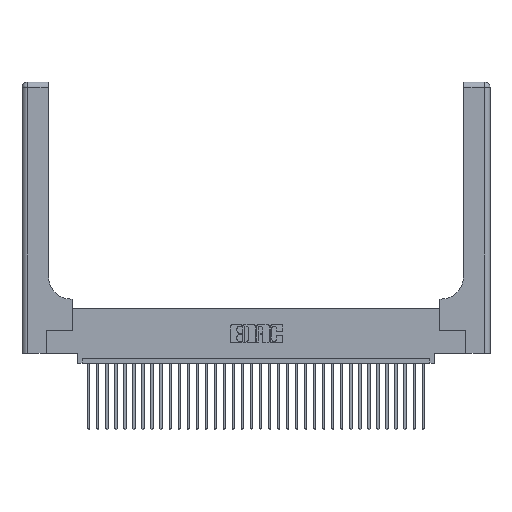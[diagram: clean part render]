
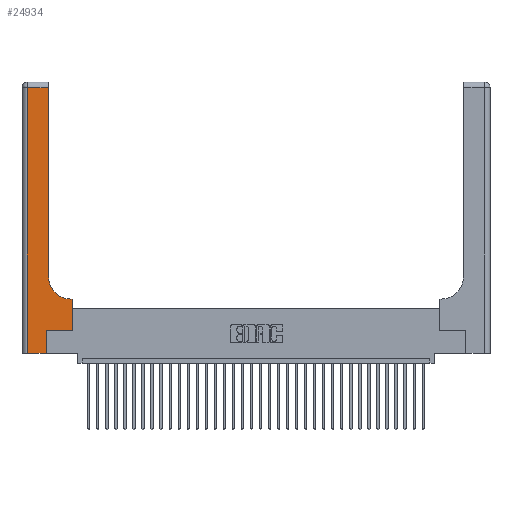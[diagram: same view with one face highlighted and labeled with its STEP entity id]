
A CAD part, top view. The second image highlights one B-rep face of the part: STEP entity #24934.
In plain terms, the highlighted planar face has unit normal (0, 0, 1).
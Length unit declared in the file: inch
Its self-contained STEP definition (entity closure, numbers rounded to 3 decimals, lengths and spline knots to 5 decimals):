
#154 = EDGE_CURVE ( 'NONE', #21570, #16127, #9224, .T. ) ;
#221 = DIRECTION ( 'NONE',  ( 1., 0., 0. ) ) ;
#1286 = CARTESIAN_POINT ( 'NONE',  ( 0.5585, 0.25, 0.37 ) ) ;
#1710 = DIRECTION ( 'NONE',  ( 0., -1., 0. ) ) ;
#2598 = LINE ( 'NONE', #5980, #32109 ) ;
#3594 = EDGE_CURVE ( 'NONE', #24266, #9584, #24757, .T. ) ;
#4675 = ORIENTED_EDGE ( 'NONE', *, *, #27138, .T. ) ;
#5340 = CARTESIAN_POINT ( 'NONE',  ( 0.269, 0.25, 0.37 ) ) ;
#5580 = CARTESIAN_POINT ( 'NONE',  ( 0.5415, 0.85, 0.37 ) ) ;
#5738 = VECTOR ( 'NONE', #5761, 39.37008 ) ;
#5761 = DIRECTION ( 'NONE',  ( 1., 0., 0. ) ) ;
#5980 = CARTESIAN_POINT ( 'NONE',  ( 0., 2.94, 0.37 ) ) ;
#6975 = VECTOR ( 'NONE', #34010, 39.37008 ) ;
#7863 = ORIENTED_EDGE ( 'NONE', *, *, #18784, .T. ) ;
#8684 = AXIS2_PLACEMENT_3D ( 'NONE', #11112, #29748, #29986 ) ;
#8697 = DIRECTION ( 'NONE',  ( 0., 0., -1. ) ) ;
#8707 = EDGE_CURVE ( 'NONE', #16127, #24266, #9422, .T. ) ;
#8940 = ORIENTED_EDGE ( 'NONE', *, *, #33445, .T. ) ;
#9014 = AXIS2_PLACEMENT_3D ( 'NONE', #5580, #8697, #221 ) ;
#9154 = CARTESIAN_POINT ( 'NONE',  ( 0.269, 0., 0.37 ) ) ;
#9224 = LINE ( 'NONE', #1286, #30463 ) ;
#9422 = LINE ( 'NONE', #27521, #29785 ) ;
#9584 = VERTEX_POINT ( 'NONE', #18418 ) ;
#11112 = CARTESIAN_POINT ( 'NONE',  ( 0., 3., 0.37 ) ) ;
#11221 = ORIENTED_EDGE ( 'NONE', *, *, #30206, .T. ) ;
#11396 = CARTESIAN_POINT ( 'NONE',  ( 0.5415, 0.6, 0.37 ) ) ;
#11425 = DIRECTION ( 'NONE',  ( -1., 0., 0. ) ) ;
#11438 = CARTESIAN_POINT ( 'NONE',  ( 0.2915, 2.94, 0.37 ) ) ;
#13589 = CARTESIAN_POINT ( 'NONE',  ( 0.2915, 3., 0.37 ) ) ;
#13590 = EDGE_CURVE ( 'NONE', #15909, #21570, #17834, .T. ) ;
#13666 = CARTESIAN_POINT ( 'NONE',  ( 0.269, 0.25, 0.37 ) ) ;
#14011 = LINE ( 'NONE', #13589, #6975 ) ;
#15769 = DIRECTION ( 'NONE',  ( 0., 1., 0. ) ) ;
#15810 = CARTESIAN_POINT ( 'NONE',  ( 0.06, 0., 0.37 ) ) ;
#15909 = VERTEX_POINT ( 'NONE', #5340 ) ;
#16071 = ORIENTED_EDGE ( 'NONE', *, *, #154, .T. ) ;
#16127 = VERTEX_POINT ( 'NONE', #21153 ) ;
#16773 = DIRECTION ( 'NONE',  ( -1., 0., 0. ) ) ;
#17480 = ORIENTED_EDGE ( 'NONE', *, *, #13590, .T. ) ;
#17834 = LINE ( 'NONE', #13666, #5738 ) ;
#18418 = CARTESIAN_POINT ( 'NONE',  ( 0.2915, 0.85, 0.37 ) ) ;
#18691 = CARTESIAN_POINT ( 'NONE',  ( 0.5585, 0.25, 0.37 ) ) ;
#18784 = EDGE_CURVE ( 'NONE', #23771, #28457, #2598, .T. ) ;
#19118 = VECTOR ( 'NONE', #15769, 39.37008 ) ;
#20869 = EDGE_CURVE ( 'NONE', #28652, #15909, #32092, .T. ) ;
#21153 = CARTESIAN_POINT ( 'NONE',  ( 0.5585, 0.6, 0.37 ) ) ;
#21570 = VERTEX_POINT ( 'NONE', #18691 ) ;
#22500 = EDGE_LOOP ( 'NONE', ( #8940, #7863, #11221, #4675, #31998, #17480, #16071, #22755, #31070 ) ) ;
#22755 = ORIENTED_EDGE ( 'NONE', *, *, #8707, .T. ) ;
#23032 = CARTESIAN_POINT ( 'NONE',  ( 0.06, 3., 0.37 ) ) ;
#23771 = VERTEX_POINT ( 'NONE', #11438 ) ;
#24266 = VERTEX_POINT ( 'NONE', #11396 ) ;
#24439 = CARTESIAN_POINT ( 'NONE',  ( 0.06, 2.94, 0.37 ) ) ;
#24736 = VERTEX_POINT ( 'NONE', #15810 ) ;
#24757 = CIRCLE ( 'NONE', #9014, 0.25 ) ;
#24934 = ADVANCED_FACE ( 'NONE', ( #29692 ), #27300, .F. ) ;
#25077 = DIRECTION ( 'NONE',  ( 0., 1., 0. ) ) ;
#26659 = CARTESIAN_POINT ( 'NONE',  ( 0., 0., 0.37 ) ) ;
#26871 = VECTOR ( 'NONE', #1710, 39.37008 ) ;
#27138 = EDGE_CURVE ( 'NONE', #24736, #28652, #32529, .T. ) ;
#27300 = PLANE ( 'NONE',  #8684 ) ;
#27509 = VECTOR ( 'NONE', #32127, 39.37008 ) ;
#27521 = CARTESIAN_POINT ( 'NONE',  ( 0.2915, 0.6, 0.37 ) ) ;
#28092 = CARTESIAN_POINT ( 'NONE',  ( 0.269, 0., 0.37 ) ) ;
#28457 = VERTEX_POINT ( 'NONE', #24439 ) ;
#28652 = VERTEX_POINT ( 'NONE', #28092 ) ;
#29692 = FACE_OUTER_BOUND ( 'NONE', #22500, .T. ) ;
#29748 = DIRECTION ( 'NONE',  ( 0., 0., -1. ) ) ;
#29785 = VECTOR ( 'NONE', #16773, 39.37008 ) ;
#29986 = DIRECTION ( 'NONE',  ( -1., 0., 0. ) ) ;
#30186 = LINE ( 'NONE', #23032, #26871 ) ;
#30206 = EDGE_CURVE ( 'NONE', #28457, #24736, #30186, .T. ) ;
#30463 = VECTOR ( 'NONE', #25077, 39.37008 ) ;
#31070 = ORIENTED_EDGE ( 'NONE', *, *, #3594, .T. ) ;
#31998 = ORIENTED_EDGE ( 'NONE', *, *, #20869, .T. ) ;
#32092 = LINE ( 'NONE', #9154, #19118 ) ;
#32109 = VECTOR ( 'NONE', #11425, 39.37008 ) ;
#32127 = DIRECTION ( 'NONE',  ( 1., 0., 0. ) ) ;
#32529 = LINE ( 'NONE', #26659, #27509 ) ;
#33445 = EDGE_CURVE ( 'NONE', #9584, #23771, #14011, .T. ) ;
#34010 = DIRECTION ( 'NONE',  ( 0., 1., 0. ) ) ;
